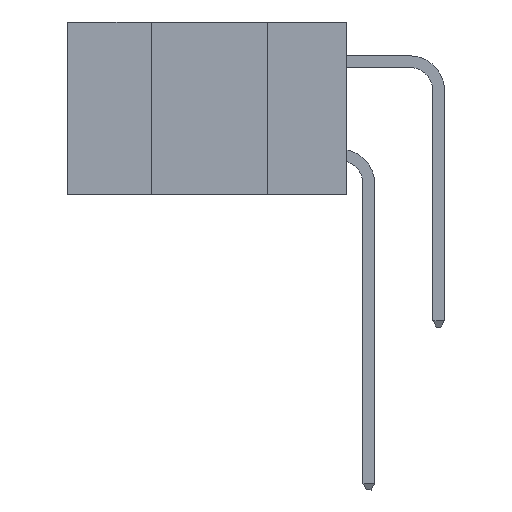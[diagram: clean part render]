
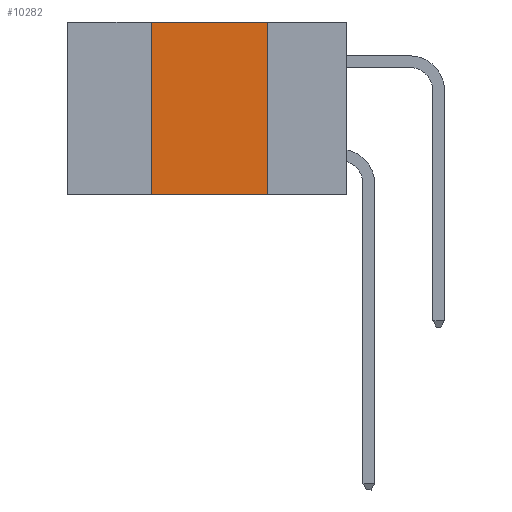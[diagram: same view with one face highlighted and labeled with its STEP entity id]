
A CAD part, left-side view. The second image highlights one B-rep face of the part: STEP entity #10282.
In plain terms, the highlighted planar face has unit normal (-1, 0, 0).
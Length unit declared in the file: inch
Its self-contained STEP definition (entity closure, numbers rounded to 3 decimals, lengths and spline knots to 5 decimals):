
#52 = EDGE_CURVE ( 'NONE', #2934, #15147, #18724, .T. ) ;
#111 = ORIENTED_EDGE ( 'NONE', *, *, #21407, .F. ) ;
#616 = CARTESIAN_POINT ( 'NONE',  ( 0., 0.42, 0. ) ) ;
#865 = PLANE ( 'NONE',  #11114 ) ;
#999 = FACE_OUTER_BOUND ( 'NONE', #8093, .T. ) ;
#2934 = VERTEX_POINT ( 'NONE', #9105 ) ;
#3366 = ORIENTED_EDGE ( 'NONE', *, *, #10572, .T. ) ;
#4583 = CARTESIAN_POINT ( 'NONE',  ( 0., 0.6, 0. ) ) ;
#6417 = VERTEX_POINT ( 'NONE', #16459 ) ;
#7349 = CARTESIAN_POINT ( 'NONE',  ( 0., 0.6, 0. ) ) ;
#8093 = EDGE_LOOP ( 'NONE', ( #111, #17989, #19672, #3366 ) ) ;
#8682 = DIRECTION ( 'NONE',  ( 0., 0., 1. ) ) ;
#8839 = VECTOR ( 'NONE', #8682, 39.37008 ) ;
#8868 = CARTESIAN_POINT ( 'NONE',  ( 0., 0.17, 0. ) ) ;
#9075 = DIRECTION ( 'NONE',  ( 0., 0., -1. ) ) ;
#9105 = CARTESIAN_POINT ( 'NONE',  ( 0., 0.42, -0.37 ) ) ;
#9766 = VECTOR ( 'NONE', #21404, 39.37008 ) ;
#10282 = ADVANCED_FACE ( 'NONE', ( #999 ), #865, .F. ) ;
#10572 = EDGE_CURVE ( 'NONE', #2934, #6417, #23717, .T. ) ;
#11114 = AXIS2_PLACEMENT_3D ( 'NONE', #4583, #18861, #9075 ) ;
#11172 = DIRECTION ( 'NONE',  ( 0., -1., 0. ) ) ;
#13343 = LINE ( 'NONE', #8868, #9766 ) ;
#13379 = CARTESIAN_POINT ( 'NONE',  ( 0., 0.42, 0. ) ) ;
#14603 = EDGE_CURVE ( 'NONE', #15147, #24477, #15004, .T. ) ;
#15004 = LINE ( 'NONE', #7349, #22979 ) ;
#15147 = VERTEX_POINT ( 'NONE', #13379 ) ;
#16459 = CARTESIAN_POINT ( 'NONE',  ( 0., 0.17, -0.37 ) ) ;
#17385 = CARTESIAN_POINT ( 'NONE',  ( 0., 0.6, -0.37 ) ) ;
#17989 = ORIENTED_EDGE ( 'NONE', *, *, #14603, .F. ) ;
#18724 = LINE ( 'NONE', #616, #8839 ) ;
#18861 = DIRECTION ( 'NONE',  ( 1., 0., 0. ) ) ;
#19009 = CARTESIAN_POINT ( 'NONE',  ( 0., 0.17, 0. ) ) ;
#19672 = ORIENTED_EDGE ( 'NONE', *, *, #52, .F. ) ;
#19794 = DIRECTION ( 'NONE',  ( 0., -1., 0. ) ) ;
#21404 = DIRECTION ( 'NONE',  ( 0., 0., -1. ) ) ;
#21407 = EDGE_CURVE ( 'NONE', #24477, #6417, #13343, .T. ) ;
#22979 = VECTOR ( 'NONE', #11172, 39.37008 ) ;
#23717 = LINE ( 'NONE', #17385, #24195 ) ;
#24195 = VECTOR ( 'NONE', #19794, 39.37008 ) ;
#24477 = VERTEX_POINT ( 'NONE', #19009 ) ;
